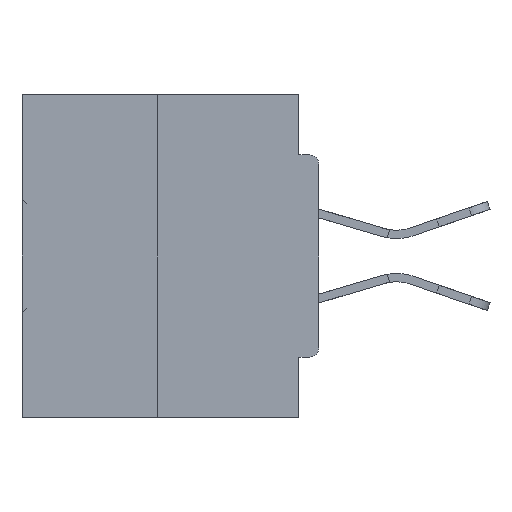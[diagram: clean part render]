
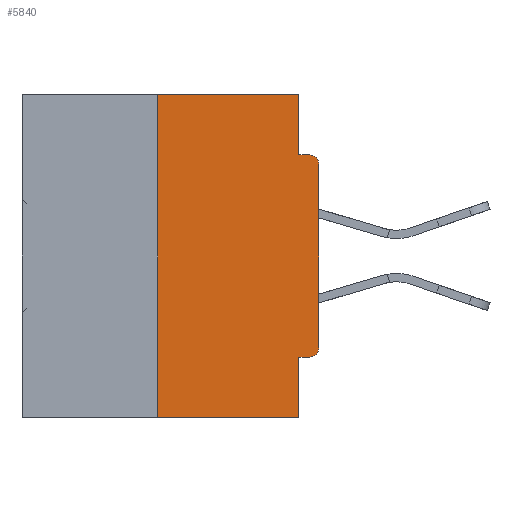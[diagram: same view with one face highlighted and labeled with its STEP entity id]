
A CAD part, left-side view. The second image highlights one B-rep face of the part: STEP entity #5840.
In plain terms, the highlighted planar face has unit normal (-1, 0, 0).
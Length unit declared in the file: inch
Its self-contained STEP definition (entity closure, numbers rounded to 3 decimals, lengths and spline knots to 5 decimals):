
#236 = DIRECTION ( 'NONE',  ( 0., -1., 0. ) ) ;
#465 = CARTESIAN_POINT ( 'NONE',  ( 0., 0.015, -0.3915 ) ) ;
#779 = CARTESIAN_POINT ( 'NONE',  ( 0., 0.25, -0.5 ) ) ;
#1061 = CARTESIAN_POINT ( 'NONE',  ( 0., 0., -0.3915 ) ) ;
#1197 = LINE ( 'NONE', #33031, #43269 ) ;
#1405 = DIRECTION ( 'NONE',  ( 0., 0., -1. ) ) ;
#1953 = ORIENTED_EDGE ( 'NONE', *, *, #43809, .F. ) ;
#2017 = ORIENTED_EDGE ( 'NONE', *, *, #45879, .F. ) ;
#2642 = CARTESIAN_POINT ( 'NONE',  ( 0., 0.015, -0.0935 ) ) ;
#2838 = EDGE_CURVE ( 'NONE', #39199, #31772, #46884, .T. ) ;
#5443 = VECTOR ( 'NONE', #35887, 39.37008 ) ;
#5840 = ADVANCED_FACE ( 'NONE', ( #23444 ), #19413, .F. ) ;
#6605 = LINE ( 'NONE', #32229, #5443 ) ;
#6708 = LINE ( 'NONE', #22530, #36233 ) ;
#6840 = AXIS2_PLACEMENT_3D ( 'NONE', #23230, #26433, #1405 ) ;
#9870 = CARTESIAN_POINT ( 'NONE',  ( 0., 0., -0.1085 ) ) ;
#10711 = CARTESIAN_POINT ( 'NONE',  ( 0., 0.031, -0.4065 ) ) ;
#11415 = AXIS2_PLACEMENT_3D ( 'NONE', #16118, #23629, #41539 ) ;
#12337 = CARTESIAN_POINT ( 'NONE',  ( 0., 0.25, 0. ) ) ;
#12491 = ORIENTED_EDGE ( 'NONE', *, *, #40914, .F. ) ;
#12804 = DIRECTION ( 'NONE',  ( 0., 0., 1. ) ) ;
#13138 = VERTEX_POINT ( 'NONE', #12337 ) ;
#13931 = CARTESIAN_POINT ( 'NONE',  ( 0., 0., 0. ) ) ;
#14785 = DIRECTION ( 'NONE',  ( 0., 0., -1. ) ) ;
#14939 = DIRECTION ( 'NONE',  ( -1., 0., 0. ) ) ;
#15489 = LINE ( 'NONE', #37755, #18311 ) ;
#15703 = CIRCLE ( 'NONE', #46652, 0.015 ) ;
#15827 = VERTEX_POINT ( 'NONE', #43394 ) ;
#16065 = VERTEX_POINT ( 'NONE', #30235 ) ;
#16118 = CARTESIAN_POINT ( 'NONE',  ( 0., 0.015, -0.1085 ) ) ;
#16660 = ORIENTED_EDGE ( 'NONE', *, *, #23497, .F. ) ;
#17263 = CARTESIAN_POINT ( 'NONE',  ( 0., 0.46, 0. ) ) ;
#17994 = VERTEX_POINT ( 'NONE', #1061 ) ;
#18311 = VECTOR ( 'NONE', #12804, 39.37008 ) ;
#19116 = VECTOR ( 'NONE', #35653, 39.37008 ) ;
#19413 = PLANE ( 'NONE',  #6840 ) ;
#20081 = LINE ( 'NONE', #13931, #44461 ) ;
#22355 = LINE ( 'NONE', #40935, #33661 ) ;
#22530 = CARTESIAN_POINT ( 'NONE',  ( 0., 0., -0.0935 ) ) ;
#23230 = CARTESIAN_POINT ( 'NONE',  ( 0., 0.46, 0. ) ) ;
#23444 = FACE_OUTER_BOUND ( 'NONE', #42560, .T. ) ;
#23497 = EDGE_CURVE ( 'NONE', #43277, #13138, #15489, .T. ) ;
#23629 = DIRECTION ( 'NONE',  ( -1., 0., 0. ) ) ;
#23779 = EDGE_CURVE ( 'NONE', #26199, #30935, #1197, .T. ) ;
#26199 = VERTEX_POINT ( 'NONE', #10711 ) ;
#26433 = DIRECTION ( 'NONE',  ( 1., 0., 0. ) ) ;
#27410 = VECTOR ( 'NONE', #47028, 39.37008 ) ;
#28744 = EDGE_CURVE ( 'NONE', #17994, #39199, #20081, .T. ) ;
#28985 = EDGE_CURVE ( 'NONE', #15827, #26199, #22355, .T. ) ;
#29315 = ORIENTED_EDGE ( 'NONE', *, *, #41383, .T. ) ;
#29719 = EDGE_CURVE ( 'NONE', #43277, #30935, #43236, .T. ) ;
#30204 = CARTESIAN_POINT ( 'NONE',  ( 0., 0.031, -0.0935 ) ) ;
#30235 = CARTESIAN_POINT ( 'NONE',  ( 0., 0.031, 0. ) ) ;
#30935 = VERTEX_POINT ( 'NONE', #44723 ) ;
#30959 = ORIENTED_EDGE ( 'NONE', *, *, #28985, .F. ) ;
#31041 = LINE ( 'NONE', #17263, #19116 ) ;
#31772 = VERTEX_POINT ( 'NONE', #2642 ) ;
#32229 = CARTESIAN_POINT ( 'NONE',  ( 0., 0.031, 0. ) ) ;
#33031 = CARTESIAN_POINT ( 'NONE',  ( 0., 0.031, -0.5 ) ) ;
#33661 = VECTOR ( 'NONE', #44418, 39.37008 ) ;
#35653 = DIRECTION ( 'NONE',  ( 0., -1., 0. ) ) ;
#35847 = DIRECTION ( 'NONE',  ( 0., 0., 1. ) ) ;
#35887 = DIRECTION ( 'NONE',  ( 0., 0., -1. ) ) ;
#36233 = VECTOR ( 'NONE', #236, 39.37008 ) ;
#36573 = CARTESIAN_POINT ( 'NONE',  ( 0., 0.46, -0.5 ) ) ;
#37755 = CARTESIAN_POINT ( 'NONE',  ( 0., 0.25, 0. ) ) ;
#38850 = ORIENTED_EDGE ( 'NONE', *, *, #28744, .T. ) ;
#39199 = VERTEX_POINT ( 'NONE', #9870 ) ;
#40098 = ORIENTED_EDGE ( 'NONE', *, *, #2838, .T. ) ;
#40365 = ORIENTED_EDGE ( 'NONE', *, *, #23779, .F. ) ;
#40914 = EDGE_CURVE ( 'NONE', #16065, #43177, #6605, .T. ) ;
#40935 = CARTESIAN_POINT ( 'NONE',  ( 0., 0., -0.4065 ) ) ;
#41383 = EDGE_CURVE ( 'NONE', #15827, #17994, #15703, .T. ) ;
#41539 = DIRECTION ( 'NONE',  ( 0., 0., -1. ) ) ;
#42560 = EDGE_LOOP ( 'NONE', ( #2017, #16660, #44268, #40365, #30959, #29315, #38850, #40098, #1953, #12491 ) ) ;
#43177 = VERTEX_POINT ( 'NONE', #30204 ) ;
#43236 = LINE ( 'NONE', #36573, #27410 ) ;
#43269 = VECTOR ( 'NONE', #43837, 39.37008 ) ;
#43277 = VERTEX_POINT ( 'NONE', #779 ) ;
#43394 = CARTESIAN_POINT ( 'NONE',  ( 0., 0.015, -0.4065 ) ) ;
#43809 = EDGE_CURVE ( 'NONE', #43177, #31772, #6708, .T. ) ;
#43837 = DIRECTION ( 'NONE',  ( 0., 0., -1. ) ) ;
#44268 = ORIENTED_EDGE ( 'NONE', *, *, #29719, .T. ) ;
#44418 = DIRECTION ( 'NONE',  ( 0., 1., 0. ) ) ;
#44461 = VECTOR ( 'NONE', #35847, 39.37008 ) ;
#44723 = CARTESIAN_POINT ( 'NONE',  ( 0., 0.031, -0.5 ) ) ;
#45879 = EDGE_CURVE ( 'NONE', #13138, #16065, #31041, .T. ) ;
#46652 = AXIS2_PLACEMENT_3D ( 'NONE', #465, #14939, #14785 ) ;
#46884 = CIRCLE ( 'NONE', #11415, 0.015 ) ;
#47028 = DIRECTION ( 'NONE',  ( 0., -1., 0. ) ) ;
